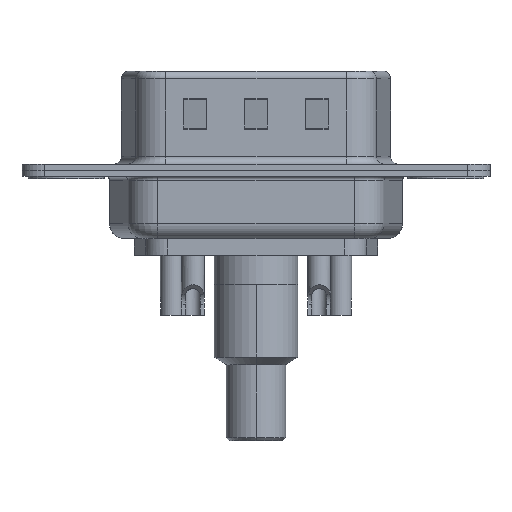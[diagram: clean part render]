
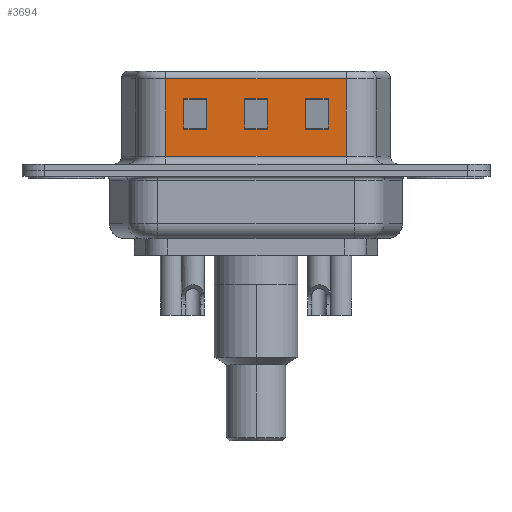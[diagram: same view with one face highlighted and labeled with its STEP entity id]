
A CAD part, front view. The second image highlights one B-rep face of the part: STEP entity #3694.
In plain terms, the highlighted planar face has unit normal (0, -1, 0).
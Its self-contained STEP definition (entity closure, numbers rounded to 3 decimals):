
#8 = ORIENTED_EDGE ( 'NONE', *, *, #4214, .T. ) ;
#175 = CARTESIAN_POINT ( 'NONE',  ( 11.75, -4.58, 2.705 ) ) ;
#233 = VERTEX_POINT ( 'NONE', #175 ) ;
#271 = VERTEX_POINT ( 'NONE', #4942 ) ;
#302 = LINE ( 'NONE', #4809, #6238 ) ;
#559 = CARTESIAN_POINT ( 'NONE',  ( 22.45, -4.58, 2.705 ) ) ;
#628 = ORIENTED_EDGE ( 'NONE', *, *, #4194, .T. ) ;
#642 = CARTESIAN_POINT ( 'NONE',  ( 15.75, -4.58, 6.52 ) ) ;
#781 = EDGE_CURVE ( 'NONE', #14101, #801, #10135, .T. ) ;
#801 = VERTEX_POINT ( 'NONE', #3912 ) ;
#855 = VERTEX_POINT ( 'NONE', #4278 ) ;
#926 = ORIENTED_EDGE ( 'NONE', *, *, #15300, .T. ) ;
#1019 = EDGE_CURVE ( 'NONE', #9522, #14101, #14643, .T. ) ;
#1260 = CARTESIAN_POINT ( 'NONE',  ( 15.75, -4.58, 4.705 ) ) ;
#1338 = DIRECTION ( 'NONE',  ( 1., 0., 0. ) ) ;
#1339 = LINE ( 'NONE', #4116, #13728 ) ;
#1380 = CARTESIAN_POINT ( 'NONE',  ( 6.55, -4.58, 0.9 ) ) ;
#1638 = CARTESIAN_POINT ( 'NONE',  ( 7.75, -4.58, 4.705 ) ) ;
#1734 = CARTESIAN_POINT ( 'NONE',  ( 13.25, -4.58, 4.705 ) ) ;
#1799 = EDGE_CURVE ( 'NONE', #11670, #9522, #13480, .T. ) ;
#1888 = DIRECTION ( 'NONE',  ( 0., 0., 1. ) ) ;
#1919 = EDGE_CURVE ( 'NONE', #801, #11670, #11634, .T. ) ;
#1950 = ORIENTED_EDGE ( 'NONE', *, *, #2827, .T. ) ;
#2165 = VERTEX_POINT ( 'NONE', #10378 ) ;
#2537 = DIRECTION ( 'NONE',  ( -1., 0., 0. ) ) ;
#2562 = CARTESIAN_POINT ( 'NONE',  ( 18.45, -4.58, 6.02 ) ) ;
#2577 = CARTESIAN_POINT ( 'NONE',  ( 11.75, -4.58, 6.52 ) ) ;
#2701 = VERTEX_POINT ( 'NONE', #1380 ) ;
#2827 = EDGE_CURVE ( 'NONE', #15451, #2165, #9928, .T. ) ;
#2841 = ORIENTED_EDGE ( 'NONE', *, *, #14727, .T. ) ;
#3009 = LINE ( 'NONE', #5008, #11087 ) ;
#3153 = FACE_BOUND ( 'NONE', #11351, .T. ) ;
#3207 = EDGE_LOOP ( 'NONE', ( #11390, #8, #628, #1950 ) ) ;
#3221 = DIRECTION ( 'NONE',  ( 0., 0., -1. ) ) ;
#3245 = DIRECTION ( 'NONE',  ( -1., 0., 0. ) ) ;
#3471 = VECTOR ( 'NONE', #12616, 1000. ) ;
#3519 = VERTEX_POINT ( 'NONE', #8047 ) ;
#3694 = ADVANCED_FACE ( 'NONE', ( #6249, #9497, #3153, #15544 ), #15457, .F. ) ;
#3912 = CARTESIAN_POINT ( 'NONE',  ( 17.25, -4.58, 4.705 ) ) ;
#4010 = CARTESIAN_POINT ( 'NONE',  ( 18.45, -4.58, 0.9 ) ) ;
#4116 = CARTESIAN_POINT ( 'NONE',  ( 18.45, -4.58, 6.52 ) ) ;
#4194 = EDGE_CURVE ( 'NONE', #271, #15451, #9885, .T. ) ;
#4214 = EDGE_CURVE ( 'NONE', #12019, #271, #302, .T. ) ;
#4277 = VECTOR ( 'NONE', #11515, 1000. ) ;
#4278 = CARTESIAN_POINT ( 'NONE',  ( 11.75, -4.58, 4.705 ) ) ;
#4283 = LINE ( 'NONE', #7507, #7412 ) ;
#4402 = EDGE_CURVE ( 'NONE', #2165, #12019, #10060, .T. ) ;
#4809 = CARTESIAN_POINT ( 'NONE',  ( 14.45, -4.58, 2.705 ) ) ;
#4891 = LINE ( 'NONE', #8380, #14138 ) ;
#4942 = CARTESIAN_POINT ( 'NONE',  ( 7.75, -4.58, 2.705 ) ) ;
#5008 = CARTESIAN_POINT ( 'NONE',  ( 18.45, -4.58, 2.705 ) ) ;
#5175 = VECTOR ( 'NONE', #3221, 1000. ) ;
#5197 = CARTESIAN_POINT ( 'NONE',  ( 6.55, -4.58, 6.52 ) ) ;
#5301 = DIRECTION ( 'NONE',  ( 1., 0., 0. ) ) ;
#5481 = CARTESIAN_POINT ( 'NONE',  ( 18.45, -4.58, 0.9 ) ) ;
#5708 = DIRECTION ( 'NONE',  ( 0., 1., 0. ) ) ;
#5827 = CARTESIAN_POINT ( 'NONE',  ( 14.45, -4.58, 4.705 ) ) ;
#5916 = DIRECTION ( 'NONE',  ( 0., 0., -1. ) ) ;
#6221 = ORIENTED_EDGE ( 'NONE', *, *, #1019, .T. ) ;
#6238 = VECTOR ( 'NONE', #2537, 1000. ) ;
#6249 = FACE_BOUND ( 'NONE', #3207, .T. ) ;
#6375 = EDGE_CURVE ( 'NONE', #14155, #3519, #4891, .T. ) ;
#6408 = VECTOR ( 'NONE', #5916, 1000. ) ;
#6517 = EDGE_CURVE ( 'NONE', #3519, #2701, #12640, .T. ) ;
#6590 = VECTOR ( 'NONE', #1888, 1000. ) ;
#6630 = VECTOR ( 'NONE', #1338, 1000. ) ;
#6646 = DIRECTION ( 'NONE',  ( 1., 0., 0. ) ) ;
#7374 = ORIENTED_EDGE ( 'NONE', *, *, #14670, .T. ) ;
#7412 = VECTOR ( 'NONE', #14800, 1000. ) ;
#7507 = CARTESIAN_POINT ( 'NONE',  ( 13.25, -4.58, 6.52 ) ) ;
#7582 = CARTESIAN_POINT ( 'NONE',  ( 9.25, -4.58, 2.705 ) ) ;
#7650 = CARTESIAN_POINT ( 'NONE',  ( 9.25, -4.58, 6.52 ) ) ;
#7773 = VECTOR ( 'NONE', #13385, 1000. ) ;
#8047 = CARTESIAN_POINT ( 'NONE',  ( 6.55, -4.58, 6.02 ) ) ;
#8195 = VECTOR ( 'NONE', #15107, 1000. ) ;
#8380 = CARTESIAN_POINT ( 'NONE',  ( 18.45, -4.58, 6.02 ) ) ;
#8410 = VERTEX_POINT ( 'NONE', #14361 ) ;
#8732 = VECTOR ( 'NONE', #5301, 1000. ) ;
#8884 = DIRECTION ( 'NONE',  ( 1., 0., 0. ) ) ;
#9061 = ORIENTED_EDGE ( 'NONE', *, *, #1919, .T. ) ;
#9073 = CARTESIAN_POINT ( 'NONE',  ( 22.45, -4.58, 4.705 ) ) ;
#9173 = CARTESIAN_POINT ( 'NONE',  ( 17.25, -4.58, 6.52 ) ) ;
#9497 = FACE_BOUND ( 'NONE', #11555, .T. ) ;
#9522 = VERTEX_POINT ( 'NONE', #12017 ) ;
#9633 = AXIS2_PLACEMENT_3D ( 'NONE', #11585, #5708, #11993 ) ;
#9885 = LINE ( 'NONE', #14736, #6590 ) ;
#9928 = LINE ( 'NONE', #5827, #6630 ) ;
#10060 = LINE ( 'NONE', #7650, #6408 ) ;
#10135 = LINE ( 'NONE', #9073, #13319 ) ;
#10378 = CARTESIAN_POINT ( 'NONE',  ( 9.25, -4.58, 4.705 ) ) ;
#10625 = LINE ( 'NONE', #5481, #13058 ) ;
#10944 = ORIENTED_EDGE ( 'NONE', *, *, #6517, .T. ) ;
#11074 = LINE ( 'NONE', #2577, #7773 ) ;
#11087 = VECTOR ( 'NONE', #12274, 1000. ) ;
#11163 = ORIENTED_EDGE ( 'NONE', *, *, #781, .T. ) ;
#11286 = EDGE_CURVE ( 'NONE', #2701, #11998, #10625, .T. ) ;
#11314 = ORIENTED_EDGE ( 'NONE', *, *, #6375, .T. ) ;
#11322 = DIRECTION ( 'NONE',  ( 0., 0., -1. ) ) ;
#11351 = EDGE_LOOP ( 'NONE', ( #12894, #2841, #7374, #926 ) ) ;
#11359 = CARTESIAN_POINT ( 'NONE',  ( 18.45, -4.58, 4.705 ) ) ;
#11390 = ORIENTED_EDGE ( 'NONE', *, *, #4402, .T. ) ;
#11515 = DIRECTION ( 'NONE',  ( -1., 0., 0. ) ) ;
#11555 = EDGE_LOOP ( 'NONE', ( #9061, #12510, #6221, #11163 ) ) ;
#11585 = CARTESIAN_POINT ( 'NONE',  ( 18.45, -4.58, 6.52 ) ) ;
#11634 = LINE ( 'NONE', #9173, #5175 ) ;
#11670 = VERTEX_POINT ( 'NONE', #11813 ) ;
#11813 = CARTESIAN_POINT ( 'NONE',  ( 17.25, -4.58, 2.705 ) ) ;
#11928 = ORIENTED_EDGE ( 'NONE', *, *, #11286, .T. ) ;
#11993 = DIRECTION ( 'NONE',  ( 0., 0., 1. ) ) ;
#11998 = VERTEX_POINT ( 'NONE', #4010 ) ;
#11999 = LINE ( 'NONE', #11359, #8732 ) ;
#12017 = CARTESIAN_POINT ( 'NONE',  ( 15.75, -4.58, 2.705 ) ) ;
#12019 = VERTEX_POINT ( 'NONE', #7582 ) ;
#12274 = DIRECTION ( 'NONE',  ( -1., 0., 0. ) ) ;
#12510 = ORIENTED_EDGE ( 'NONE', *, *, #1799, .T. ) ;
#12616 = DIRECTION ( 'NONE',  ( 0., 0., -1. ) ) ;
#12640 = LINE ( 'NONE', #5197, #3471 ) ;
#12894 = ORIENTED_EDGE ( 'NONE', *, *, #15501, .T. ) ;
#13058 = VECTOR ( 'NONE', #6646, 1000. ) ;
#13141 = EDGE_CURVE ( 'NONE', #14155, #11998, #1339, .T. ) ;
#13319 = VECTOR ( 'NONE', #8884, 1000. ) ;
#13385 = DIRECTION ( 'NONE',  ( 0., 0., 1. ) ) ;
#13480 = LINE ( 'NONE', #559, #4277 ) ;
#13728 = VECTOR ( 'NONE', #11322, 1000. ) ;
#13740 = EDGE_LOOP ( 'NONE', ( #14118, #11314, #10944, #11928 ) ) ;
#14101 = VERTEX_POINT ( 'NONE', #1260 ) ;
#14118 = ORIENTED_EDGE ( 'NONE', *, *, #13141, .F. ) ;
#14138 = VECTOR ( 'NONE', #3245, 1000. ) ;
#14155 = VERTEX_POINT ( 'NONE', #2562 ) ;
#14361 = CARTESIAN_POINT ( 'NONE',  ( 13.25, -4.58, 2.705 ) ) ;
#14643 = LINE ( 'NONE', #642, #8195 ) ;
#14670 = EDGE_CURVE ( 'NONE', #8410, #233, #3009, .T. ) ;
#14727 = EDGE_CURVE ( 'NONE', #15467, #8410, #4283, .T. ) ;
#14736 = CARTESIAN_POINT ( 'NONE',  ( 7.75, -4.58, 6.52 ) ) ;
#14800 = DIRECTION ( 'NONE',  ( 0., 0., -1. ) ) ;
#15107 = DIRECTION ( 'NONE',  ( 0., 0., 1. ) ) ;
#15300 = EDGE_CURVE ( 'NONE', #233, #855, #11074, .T. ) ;
#15451 = VERTEX_POINT ( 'NONE', #1638 ) ;
#15457 = PLANE ( 'NONE',  #9633 ) ;
#15467 = VERTEX_POINT ( 'NONE', #1734 ) ;
#15501 = EDGE_CURVE ( 'NONE', #855, #15467, #11999, .T. ) ;
#15544 = FACE_OUTER_BOUND ( 'NONE', #13740, .T. ) ;
